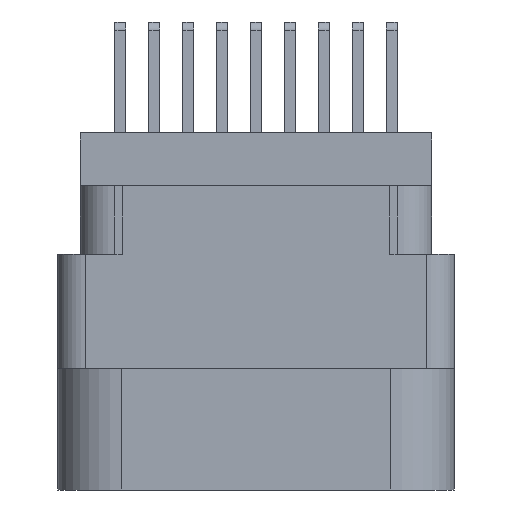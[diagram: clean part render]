
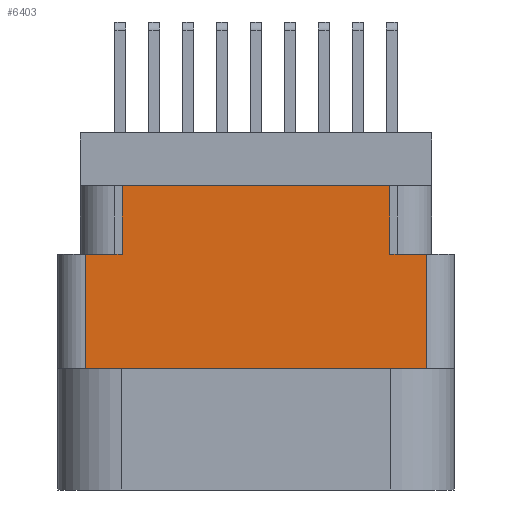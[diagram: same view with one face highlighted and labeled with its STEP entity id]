
A CAD part, left-side view. The second image highlights one B-rep face of the part: STEP entity #6403.
In plain terms, the highlighted planar face has unit normal (-1, 0, 0).
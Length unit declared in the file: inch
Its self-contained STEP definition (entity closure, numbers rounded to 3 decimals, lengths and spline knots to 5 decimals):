
#1138 = ORIENTED_EDGE ( 'NONE', *, *, #8640, .T. ) ;
#1678 = LINE ( 'NONE', #10805, #22468 ) ;
#1948 = VERTEX_POINT ( 'NONE', #12581 ) ;
#2643 = CARTESIAN_POINT ( 'NONE',  ( -1., -0.376, -0.789 ) ) ;
#2749 = CARTESIAN_POINT ( 'NONE',  ( -1., -0.296, -0.268 ) ) ;
#3133 = CARTESIAN_POINT ( 'NONE',  ( -1., 0., -0.268 ) ) ;
#3184 = CARTESIAN_POINT ( 'NONE',  ( -1., 0.376, -0.789 ) ) ;
#3708 = ORIENTED_EDGE ( 'NONE', *, *, #23844, .T. ) ;
#3998 = LINE ( 'NONE', #2749, #31762 ) ;
#4301 = ORIENTED_EDGE ( 'NONE', *, *, #30909, .F. ) ;
#4351 = CARTESIAN_POINT ( 'NONE',  ( -1., 0., -0.52 ) ) ;
#4638 = PLANE ( 'NONE',  #14552 ) ;
#4660 = ORIENTED_EDGE ( 'NONE', *, *, #17854, .T. ) ;
#5495 = VECTOR ( 'NONE', #12026, 39.37008 ) ;
#5996 = DIRECTION ( 'NONE',  ( 0., -1., 0. ) ) ;
#6112 = VERTEX_POINT ( 'NONE', #21826 ) ;
#6403 = ADVANCED_FACE ( 'NONE', ( #19610 ), #4638, .T. ) ;
#6633 = VERTEX_POINT ( 'NONE', #24417 ) ;
#6667 = CARTESIAN_POINT ( 'NONE',  ( -1., 0.296, -0.117 ) ) ;
#7125 = DIRECTION ( 'NONE',  ( -1., 0., 0. ) ) ;
#8217 = CARTESIAN_POINT ( 'NONE',  ( -1., -0.296, -0.268 ) ) ;
#8640 = EDGE_CURVE ( 'NONE', #18891, #1948, #10903, .T. ) ;
#8745 = CARTESIAN_POINT ( 'NONE',  ( -1., 0., -0.268 ) ) ;
#10186 = VECTOR ( 'NONE', #25538, 39.37008 ) ;
#10715 = DIRECTION ( 'NONE',  ( 0., 0., -1. ) ) ;
#10805 = CARTESIAN_POINT ( 'NONE',  ( -1., 0.438, -0.117 ) ) ;
#10814 = ORIENTED_EDGE ( 'NONE', *, *, #19935, .T. ) ;
#10903 = LINE ( 'NONE', #4351, #25168 ) ;
#12026 = DIRECTION ( 'NONE',  ( 0., -1., 0. ) ) ;
#12111 = CARTESIAN_POINT ( 'NONE',  ( -1., 0.296, -0.268 ) ) ;
#12581 = CARTESIAN_POINT ( 'NONE',  ( -1., -0.376, -0.52 ) ) ;
#14552 = AXIS2_PLACEMENT_3D ( 'NONE', #17493, #7125, #27884 ) ;
#15203 = VERTEX_POINT ( 'NONE', #8217 ) ;
#15684 = EDGE_CURVE ( 'NONE', #26116, #6112, #1678, .T. ) ;
#16437 = DIRECTION ( 'NONE',  ( 0., -1., 0. ) ) ;
#17493 = CARTESIAN_POINT ( 'NONE',  ( -1., -0.438, -0.789 ) ) ;
#17854 = EDGE_CURVE ( 'NONE', #1948, #6633, #18386, .T. ) ;
#18386 = LINE ( 'NONE', #2643, #24106 ) ;
#18452 = DIRECTION ( 'NONE',  ( 0., 0., 1. ) ) ;
#18891 = VERTEX_POINT ( 'NONE', #19589 ) ;
#19005 = CARTESIAN_POINT ( 'NONE',  ( -1., 0.376, -0.268 ) ) ;
#19589 = CARTESIAN_POINT ( 'NONE',  ( -1., 0.376, -0.52 ) ) ;
#19610 = FACE_OUTER_BOUND ( 'NONE', #29823, .T. ) ;
#19935 = EDGE_CURVE ( 'NONE', #15203, #6112, #3998, .T. ) ;
#20031 = ORIENTED_EDGE ( 'NONE', *, *, #26071, .F. ) ;
#20033 = VERTEX_POINT ( 'NONE', #19005 ) ;
#20141 = ORIENTED_EDGE ( 'NONE', *, *, #25501, .F. ) ;
#20833 = ORIENTED_EDGE ( 'NONE', *, *, #15684, .F. ) ;
#21303 = VECTOR ( 'NONE', #10715, 39.37008 ) ;
#21826 = CARTESIAN_POINT ( 'NONE',  ( -1., -0.296, -0.117 ) ) ;
#22468 = VECTOR ( 'NONE', #29164, 39.37008 ) ;
#23153 = DIRECTION ( 'NONE',  ( 0., 0., 1. ) ) ;
#23844 = EDGE_CURVE ( 'NONE', #20033, #18891, #30722, .T. ) ;
#24106 = VECTOR ( 'NONE', #23153, 39.37008 ) ;
#24417 = CARTESIAN_POINT ( 'NONE',  ( -1., -0.376, -0.268 ) ) ;
#25032 = LINE ( 'NONE', #3133, #25847 ) ;
#25168 = VECTOR ( 'NONE', #16437, 39.37008 ) ;
#25501 = EDGE_CURVE ( 'NONE', #15203, #6633, #32854, .T. ) ;
#25538 = DIRECTION ( 'NONE',  ( 0., 0., 1. ) ) ;
#25847 = VECTOR ( 'NONE', #5996, 39.37008 ) ;
#26071 = EDGE_CURVE ( 'NONE', #20033, #28878, #25032, .T. ) ;
#26116 = VERTEX_POINT ( 'NONE', #6667 ) ;
#27884 = DIRECTION ( 'NONE',  ( 0., 0., 1. ) ) ;
#28878 = VERTEX_POINT ( 'NONE', #33654 ) ;
#29164 = DIRECTION ( 'NONE',  ( 0., -1., 0. ) ) ;
#29823 = EDGE_LOOP ( 'NONE', ( #20031, #3708, #1138, #4660, #20141, #10814, #20833, #4301 ) ) ;
#30722 = LINE ( 'NONE', #3184, #21303 ) ;
#30909 = EDGE_CURVE ( 'NONE', #28878, #26116, #32670, .T. ) ;
#31762 = VECTOR ( 'NONE', #18452, 39.37008 ) ;
#32670 = LINE ( 'NONE', #12111, #10186 ) ;
#32854 = LINE ( 'NONE', #8745, #5495 ) ;
#33654 = CARTESIAN_POINT ( 'NONE',  ( -1., 0.296, -0.268 ) ) ;
